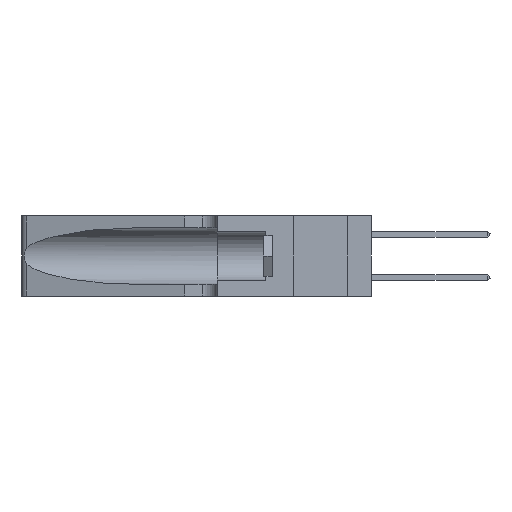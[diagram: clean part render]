
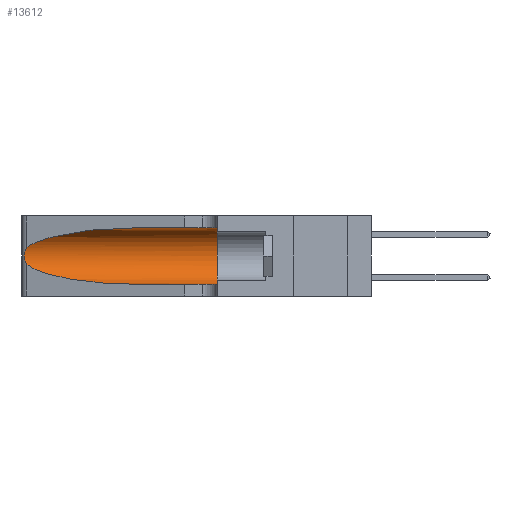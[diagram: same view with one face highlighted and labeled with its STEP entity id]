
A CAD part, left-side view. The second image highlights one B-rep face of the part: STEP entity #13612.
In plain terms, the highlighted cylindrical face has radius 3.308 mm (diameter 6.617 mm), a partial arc.
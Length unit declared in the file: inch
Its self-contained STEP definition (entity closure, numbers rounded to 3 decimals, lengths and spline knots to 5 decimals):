
#455 = FACE_OUTER_BOUND ( 'NONE', #3953, .T. ) ;
#535 = ORIENTED_EDGE ( 'NONE', *, *, #28470, .T. ) ;
#1367 = EDGE_CURVE ( 'NONE', #23626, #28316, #7827, .T. ) ;
#1566 = ORIENTED_EDGE ( 'NONE', *, *, #1367, .T. ) ;
#1956 = EDGE_CURVE ( 'NONE', #26156, #4921, #23580, .T. ) ;
#2077 = EDGE_CURVE ( 'NONE', #16823, #26156, #34533, .T. ) ;
#2734 = AXIS2_PLACEMENT_3D ( 'NONE', #25379, #14598, #3607 ) ;
#3607 = DIRECTION ( 'NONE',  ( 0., 0., -1. ) ) ;
#3680 = CARTESIAN_POINT ( 'NONE',  ( 0.1305, 0.35, 0.31525 ) ) ;
#3953 = EDGE_LOOP ( 'NONE', ( #20860, #1566, #535, #9253, #8734, #9147 ) ) ;
#4100 = CARTESIAN_POINT ( 'NONE',  ( 0.25639, 1.23186, 0.15144 ) ) ;
#4764 = CARTESIAN_POINT ( 'NONE',  ( 0.1305, 0.72297, 0.31525 ) ) ;
#4893 = CARTESIAN_POINT ( 'NONE',  ( 0.26018, 1.23835, 0.19895 ) ) ;
#4921 = VERTEX_POINT ( 'NONE', #13793 ) ;
#5960 = DIRECTION ( 'NONE',  ( 0., -1., 0. ) ) ;
#6139 = LINE ( 'NONE', #23473, #19702 ) ;
#6773 = CARTESIAN_POINT ( 'NONE',  ( 0.25856, 1.23593, 0.16098 ) ) ;
#6896 = CARTESIAN_POINT ( 'NONE',  ( 0.25854, 1.2359, 0.20912 ) ) ;
#7030 = CYLINDRICAL_SURFACE ( 'NONE', #2734, 0.13025 ) ;
#7278 = CARTESIAN_POINT ( 'NONE',  ( 0.25787, 1.23484, 0.2124 ) ) ;
#7827 = B_SPLINE_CURVE_WITH_KNOTS ( 'NONE', 3,
 ( #26466, #10086, #27738, #7278, #6896, #4893, #26152, #31694, #26621, #6773, #29934, #4100, #32158, #33767 ),
 .UNSPECIFIED., .F., .F.,
 ( 4, 2, 2, 2, 2, 2, 4 ),
 ( 0., 0.00027, 0.00053, 0.00107, 0.0016, 0.00187, 0.00214 ),
 .UNSPECIFIED. ) ;
#8239 = CARTESIAN_POINT ( 'NONE',  ( 0.1305, 0.72297, 0.05475 ) ) ;
#8734 = ORIENTED_EDGE ( 'NONE', *, *, #1956, .F. ) ;
#9147 = ORIENTED_EDGE ( 'NONE', *, *, #2077, .F. ) ;
#9253 = ORIENTED_EDGE ( 'NONE', *, *, #27629, .T. ) ;
#9826 = CARTESIAN_POINT ( 'NONE',  ( 0.25487, 1.22718, 0.22369 ) ) ;
#10086 = CARTESIAN_POINT ( 'NONE',  ( 0.25555, 1.22994, 0.2215 ) ) ;
#11051 = DIRECTION ( 'NONE',  ( 0., 1., 0. ) ) ;
#11384 = CARTESIAN_POINT ( 'NONE',  ( 0.1305, 1.61858, 0.31525 ) ) ;
#12677 = DIRECTION ( 'NONE',  ( 0., -1., 0. ) ) ;
#13612 = ADVANCED_FACE ( 'NONE', ( #455 ), #7030, .F. ) ;
#13793 = CARTESIAN_POINT ( 'NONE',  ( 0.1305, 0.35, 0.05475 ) ) ;
#14598 = DIRECTION ( 'NONE',  ( 0., -1., 0. ) ) ;
#14637 = CARTESIAN_POINT ( 'NONE',  ( 0.1305, 0.72297, 0.05475 ) ) ;
#15244 =( BOUNDED_CURVE ( )  B_SPLINE_CURVE ( 3, ( #16331, #29825, #24522, #8239 ),
 .UNSPECIFIED., .F., .F. ) 
 B_SPLINE_CURVE_WITH_KNOTS ( ( 4, 4 ),
 ( 3.44316, 4.71239 ),
 .UNSPECIFIED. ) 
 CURVE ( )  GEOMETRIC_REPRESENTATION_ITEM ( )  RATIONAL_B_SPLINE_CURVE ( ( 1., 0.87, 0.87, 1. ) ) 
 REPRESENTATION_ITEM ( '' )  );
#16253 = AXIS2_PLACEMENT_3D ( 'NONE', #27292, #11051, #30047 ) ;
#16331 = CARTESIAN_POINT ( 'NONE',  ( 0.25487, 1.22718, 0.14631 ) ) ;
#16823 = VERTEX_POINT ( 'NONE', #4764 ) ;
#19105 = CARTESIAN_POINT ( 'NONE',  ( 0.25487, 1.22718, 0.22369 ) ) ;
#19702 = VECTOR ( 'NONE', #12677, 39.37008 ) ;
#20860 = ORIENTED_EDGE ( 'NONE', *, *, #25266, .T. ) ;
#21023 = VECTOR ( 'NONE', #5960, 39.37008 ) ;
#21553 =( BOUNDED_CURVE ( )  B_SPLINE_CURVE ( 3, ( #29901, #24476, #34995, #19105 ),
 .UNSPECIFIED., .F., .F. ) 
 B_SPLINE_CURVE_WITH_KNOTS ( ( 4, 4 ),
 ( 1.5708, 2.84003 ),
 .UNSPECIFIED. ) 
 CURVE ( )  GEOMETRIC_REPRESENTATION_ITEM ( )  RATIONAL_B_SPLINE_CURVE ( ( 1., 0.87, 0.87, 1. ) ) 
 REPRESENTATION_ITEM ( '' )  );
#22690 = VERTEX_POINT ( 'NONE', #14637 ) ;
#23473 = CARTESIAN_POINT ( 'NONE',  ( 0.1305, 1.61858, 0.05475 ) ) ;
#23580 = CIRCLE ( 'NONE', #16253, 0.13025 ) ;
#23626 = VERTEX_POINT ( 'NONE', #9826 ) ;
#24476 = CARTESIAN_POINT ( 'NONE',  ( 0.18966, 0.96281, 0.31525 ) ) ;
#24522 = CARTESIAN_POINT ( 'NONE',  ( 0.18966, 0.96281, 0.05475 ) ) ;
#25266 = EDGE_CURVE ( 'NONE', #16823, #23626, #21553, .T. ) ;
#25379 = CARTESIAN_POINT ( 'NONE',  ( 0.1305, 1.61858, 0.185 ) ) ;
#26152 = CARTESIAN_POINT ( 'NONE',  ( 0.26075, 1.23896, 0.19203 ) ) ;
#26156 = VERTEX_POINT ( 'NONE', #3680 ) ;
#26466 = CARTESIAN_POINT ( 'NONE',  ( 0.25487, 1.22718, 0.22369 ) ) ;
#26621 = CARTESIAN_POINT ( 'NONE',  ( 0.26017, 1.23833, 0.17102 ) ) ;
#27292 = CARTESIAN_POINT ( 'NONE',  ( 0.1305, 0.35, 0.185 ) ) ;
#27629 = EDGE_CURVE ( 'NONE', #22690, #4921, #6139, .T. ) ;
#27738 = CARTESIAN_POINT ( 'NONE',  ( 0.25639, 1.23184, 0.21858 ) ) ;
#28316 = VERTEX_POINT ( 'NONE', #29355 ) ;
#28470 = EDGE_CURVE ( 'NONE', #28316, #22690, #15244, .T. ) ;
#29355 = CARTESIAN_POINT ( 'NONE',  ( 0.25487, 1.22718, 0.14631 ) ) ;
#29825 = CARTESIAN_POINT ( 'NONE',  ( 0.2373, 1.15595, 0.08982 ) ) ;
#29901 = CARTESIAN_POINT ( 'NONE',  ( 0.1305, 0.72297, 0.31525 ) ) ;
#29934 = CARTESIAN_POINT ( 'NONE',  ( 0.25789, 1.23486, 0.15765 ) ) ;
#30047 = DIRECTION ( 'NONE',  ( 0., 0., 1. ) ) ;
#31694 = CARTESIAN_POINT ( 'NONE',  ( 0.26075, 1.23896, 0.178 ) ) ;
#32158 = CARTESIAN_POINT ( 'NONE',  ( 0.25555, 1.22993, 0.14849 ) ) ;
#33767 = CARTESIAN_POINT ( 'NONE',  ( 0.25487, 1.22718, 0.14631 ) ) ;
#34533 = LINE ( 'NONE', #11384, #21023 ) ;
#34995 = CARTESIAN_POINT ( 'NONE',  ( 0.2373, 1.15595, 0.28018 ) ) ;
